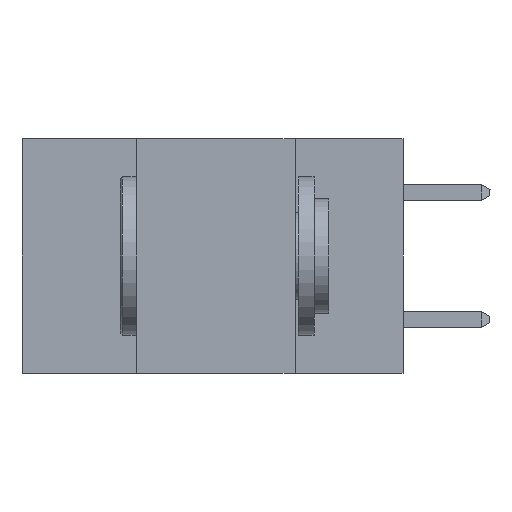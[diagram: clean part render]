
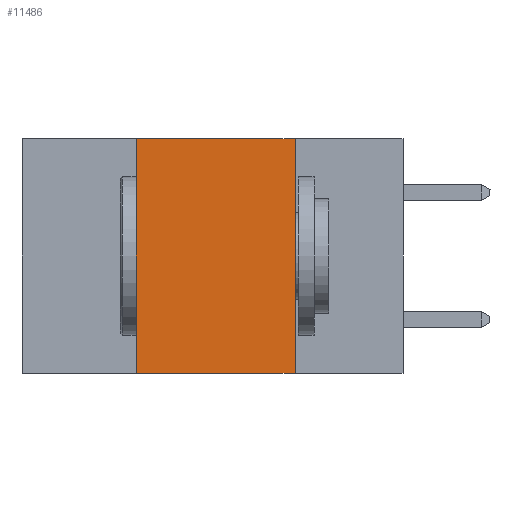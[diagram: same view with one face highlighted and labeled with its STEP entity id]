
A CAD part, left-side view. The second image highlights one B-rep face of the part: STEP entity #11486.
In plain terms, the highlighted planar face has unit normal (-1, 0, 0).
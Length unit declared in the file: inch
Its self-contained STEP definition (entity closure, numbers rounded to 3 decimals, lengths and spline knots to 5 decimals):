
#45 = EDGE_CURVE ( 'NONE', #715, #6173, #788, .T. ) ;
#408 = VECTOR ( 'NONE', #7085, 39.37008 ) ;
#628 = CARTESIAN_POINT ( 'NONE',  ( 0., 0.17, 0. ) ) ;
#715 = VERTEX_POINT ( 'NONE', #7545 ) ;
#788 = LINE ( 'NONE', #8117, #2472 ) ;
#1118 = ORIENTED_EDGE ( 'NONE', *, *, #45, .F. ) ;
#1310 = VECTOR ( 'NONE', #8144, 39.37008 ) ;
#1774 = CARTESIAN_POINT ( 'NONE',  ( 0., 0.6, 0. ) ) ;
#2472 = VECTOR ( 'NONE', #4508, 39.37008 ) ;
#2638 = CARTESIAN_POINT ( 'NONE',  ( 0., 0.17, 0. ) ) ;
#2983 = DIRECTION ( 'NONE',  ( 0., -1., 0. ) ) ;
#3243 = DIRECTION ( 'NONE',  ( 1., 0., 0. ) ) ;
#3673 = EDGE_LOOP ( 'NONE', ( #7076, #8296, #1118, #8318 ) ) ;
#3826 = LINE ( 'NONE', #1774, #1310 ) ;
#3952 = CARTESIAN_POINT ( 'NONE',  ( 0., 0.42, 0. ) ) ;
#4050 = CARTESIAN_POINT ( 'NONE',  ( 0., 0.6, -0.37 ) ) ;
#4332 = EDGE_CURVE ( 'NONE', #6173, #10361, #3826, .T. ) ;
#4508 = DIRECTION ( 'NONE',  ( 0., 0., 1. ) ) ;
#4747 = VECTOR ( 'NONE', #2983, 39.37008 ) ;
#6122 = AXIS2_PLACEMENT_3D ( 'NONE', #6900, #3243, #9565 ) ;
#6173 = VERTEX_POINT ( 'NONE', #3952 ) ;
#6581 = CARTESIAN_POINT ( 'NONE',  ( 0., 0.17, -0.37 ) ) ;
#6900 = CARTESIAN_POINT ( 'NONE',  ( 0., 0.6, 0. ) ) ;
#6938 = PLANE ( 'NONE',  #6122 ) ;
#7076 = ORIENTED_EDGE ( 'NONE', *, *, #10734, .F. ) ;
#7085 = DIRECTION ( 'NONE',  ( 0., 0., -1. ) ) ;
#7140 = LINE ( 'NONE', #4050, #4747 ) ;
#7545 = CARTESIAN_POINT ( 'NONE',  ( 0., 0.42, -0.37 ) ) ;
#8117 = CARTESIAN_POINT ( 'NONE',  ( 0., 0.42, 0. ) ) ;
#8144 = DIRECTION ( 'NONE',  ( 0., -1., 0. ) ) ;
#8296 = ORIENTED_EDGE ( 'NONE', *, *, #4332, .F. ) ;
#8318 = ORIENTED_EDGE ( 'NONE', *, *, #8336, .T. ) ;
#8336 = EDGE_CURVE ( 'NONE', #715, #10779, #7140, .T. ) ;
#9565 = DIRECTION ( 'NONE',  ( 0., 0., -1. ) ) ;
#10274 = FACE_OUTER_BOUND ( 'NONE', #3673, .T. ) ;
#10361 = VERTEX_POINT ( 'NONE', #2638 ) ;
#10734 = EDGE_CURVE ( 'NONE', #10361, #10779, #11405, .T. ) ;
#10779 = VERTEX_POINT ( 'NONE', #6581 ) ;
#11405 = LINE ( 'NONE', #628, #408 ) ;
#11486 = ADVANCED_FACE ( 'NONE', ( #10274 ), #6938, .F. ) ;
